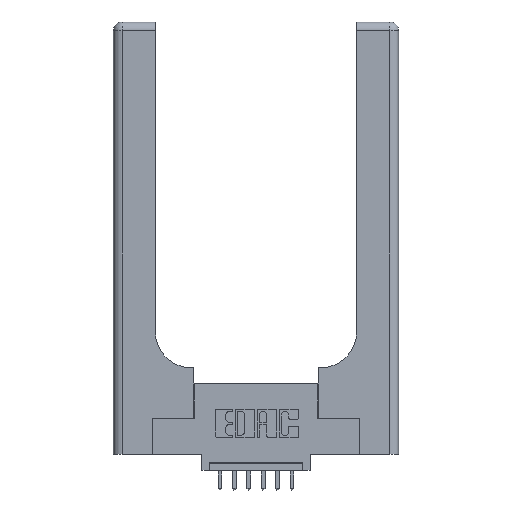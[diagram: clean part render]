
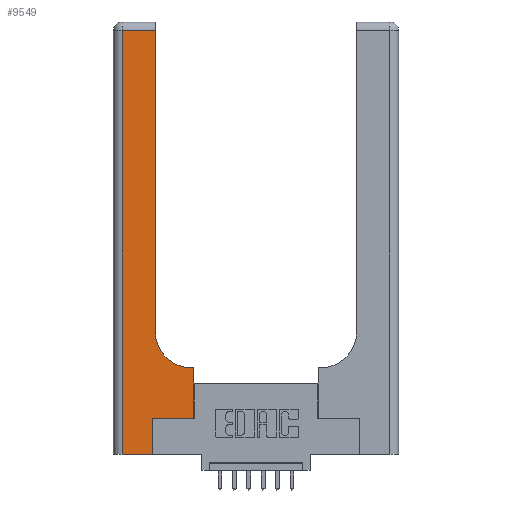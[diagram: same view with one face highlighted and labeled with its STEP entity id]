
A CAD part, top view. The second image highlights one B-rep face of the part: STEP entity #9549.
In plain terms, the highlighted planar face has unit normal (0, 0, 1).
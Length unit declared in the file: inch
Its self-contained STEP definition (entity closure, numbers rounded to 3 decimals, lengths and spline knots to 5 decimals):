
#137 = CARTESIAN_POINT ( 'NONE',  ( 0.5415, 0.85, 0.37 ) ) ;
#236 = CARTESIAN_POINT ( 'NONE',  ( 0.06, 3., 0.37 ) ) ;
#238 = EDGE_CURVE ( 'NONE', #4879, #9358, #3338, .T. ) ;
#274 = DIRECTION ( 'NONE',  ( 0., 1., 0. ) ) ;
#506 = LINE ( 'NONE', #9152, #2619 ) ;
#515 = EDGE_CURVE ( 'NONE', #2527, #6985, #2794, .T. ) ;
#614 = DIRECTION ( 'NONE',  ( -1., 0., 0. ) ) ;
#635 = LINE ( 'NONE', #14375, #2050 ) ;
#674 = DIRECTION ( 'NONE',  ( -1., 0., 0. ) ) ;
#1168 = CARTESIAN_POINT ( 'NONE',  ( 0.2915, 2.94, 0.37 ) ) ;
#1397 = CARTESIAN_POINT ( 'NONE',  ( 0.2915, 3., 0.37 ) ) ;
#1679 = ORIENTED_EDGE ( 'NONE', *, *, #5510, .T. ) ;
#1948 = ORIENTED_EDGE ( 'NONE', *, *, #238, .T. ) ;
#2050 = VECTOR ( 'NONE', #674, 39.37008 ) ;
#2288 = VERTEX_POINT ( 'NONE', #5535 ) ;
#2420 = VECTOR ( 'NONE', #274, 39.37008 ) ;
#2527 = VERTEX_POINT ( 'NONE', #14128 ) ;
#2609 = VECTOR ( 'NONE', #11451, 39.37008 ) ;
#2619 = VECTOR ( 'NONE', #3459, 39.37008 ) ;
#2646 = CARTESIAN_POINT ( 'NONE',  ( 0.269, 0.25, 0.37 ) ) ;
#2728 = CARTESIAN_POINT ( 'NONE',  ( 0.2915, 0.6, 0.37 ) ) ;
#2794 = LINE ( 'NONE', #1397, #2420 ) ;
#3338 = LINE ( 'NONE', #236, #2609 ) ;
#3459 = DIRECTION ( 'NONE',  ( 1., 0., 0. ) ) ;
#3832 = DIRECTION ( 'NONE',  ( -1., 0., 0. ) ) ;
#4016 = EDGE_CURVE ( 'NONE', #4122, #7114, #7437, .T. ) ;
#4049 = EDGE_CURVE ( 'NONE', #7114, #7739, #4609, .T. ) ;
#4122 = VERTEX_POINT ( 'NONE', #6364 ) ;
#4609 = LINE ( 'NONE', #2646, #12596 ) ;
#4657 = FACE_OUTER_BOUND ( 'NONE', #4979, .T. ) ;
#4826 = EDGE_CURVE ( 'NONE', #9358, #4122, #506, .T. ) ;
#4871 = CARTESIAN_POINT ( 'NONE',  ( 0.5585, 0.25, 0.37 ) ) ;
#4879 = VERTEX_POINT ( 'NONE', #6829 ) ;
#4979 = EDGE_LOOP ( 'NONE', ( #12961, #14615, #1948, #8082, #6424, #6780, #1679, #11192, #9993 ) ) ;
#5103 = LINE ( 'NONE', #4871, #8466 ) ;
#5209 = CIRCLE ( 'NONE', #8285, 0.25 ) ;
#5510 = EDGE_CURVE ( 'NONE', #7739, #9836, #5103, .T. ) ;
#5535 = CARTESIAN_POINT ( 'NONE',  ( 0.5415, 0.6, 0.37 ) ) ;
#6364 = CARTESIAN_POINT ( 'NONE',  ( 0.269, 0., 0.37 ) ) ;
#6424 = ORIENTED_EDGE ( 'NONE', *, *, #4016, .T. ) ;
#6780 = ORIENTED_EDGE ( 'NONE', *, *, #4049, .T. ) ;
#6829 = CARTESIAN_POINT ( 'NONE',  ( 0.06, 2.94, 0.37 ) ) ;
#6864 = CARTESIAN_POINT ( 'NONE',  ( 0.5585, 0.6, 0.37 ) ) ;
#6985 = VERTEX_POINT ( 'NONE', #1168 ) ;
#7079 = VECTOR ( 'NONE', #11590, 39.37008 ) ;
#7101 = DIRECTION ( 'NONE',  ( 0., 1., 0. ) ) ;
#7103 = LINE ( 'NONE', #2728, #12258 ) ;
#7114 = VERTEX_POINT ( 'NONE', #10440 ) ;
#7437 = LINE ( 'NONE', #12838, #7079 ) ;
#7444 = EDGE_CURVE ( 'NONE', #6985, #4879, #635, .T. ) ;
#7595 = PLANE ( 'NONE',  #8007 ) ;
#7739 = VERTEX_POINT ( 'NONE', #12479 ) ;
#8007 = AXIS2_PLACEMENT_3D ( 'NONE', #14362, #14409, #614 ) ;
#8082 = ORIENTED_EDGE ( 'NONE', *, *, #4826, .T. ) ;
#8285 = AXIS2_PLACEMENT_3D ( 'NONE', #137, #9202, #10359 ) ;
#8466 = VECTOR ( 'NONE', #7101, 39.37008 ) ;
#8974 = EDGE_CURVE ( 'NONE', #2288, #2527, #5209, .T. ) ;
#9152 = CARTESIAN_POINT ( 'NONE',  ( 0., 0., 0.37 ) ) ;
#9202 = DIRECTION ( 'NONE',  ( 0., 0., -1. ) ) ;
#9293 = CARTESIAN_POINT ( 'NONE',  ( 0.06, 0., 0.37 ) ) ;
#9358 = VERTEX_POINT ( 'NONE', #9293 ) ;
#9549 = ADVANCED_FACE ( 'NONE', ( #4657 ), #7595, .F. ) ;
#9836 = VERTEX_POINT ( 'NONE', #6864 ) ;
#9993 = ORIENTED_EDGE ( 'NONE', *, *, #8974, .T. ) ;
#10359 = DIRECTION ( 'NONE',  ( 1., 0., 0. ) ) ;
#10440 = CARTESIAN_POINT ( 'NONE',  ( 0.269, 0.25, 0.37 ) ) ;
#10508 = EDGE_CURVE ( 'NONE', #9836, #2288, #7103, .T. ) ;
#10602 = DIRECTION ( 'NONE',  ( 1., 0., 0. ) ) ;
#11192 = ORIENTED_EDGE ( 'NONE', *, *, #10508, .T. ) ;
#11451 = DIRECTION ( 'NONE',  ( 0., -1., 0. ) ) ;
#11590 = DIRECTION ( 'NONE',  ( 0., 1., 0. ) ) ;
#12258 = VECTOR ( 'NONE', #3832, 39.37008 ) ;
#12479 = CARTESIAN_POINT ( 'NONE',  ( 0.5585, 0.25, 0.37 ) ) ;
#12596 = VECTOR ( 'NONE', #10602, 39.37008 ) ;
#12838 = CARTESIAN_POINT ( 'NONE',  ( 0.269, 0., 0.37 ) ) ;
#12961 = ORIENTED_EDGE ( 'NONE', *, *, #515, .T. ) ;
#14128 = CARTESIAN_POINT ( 'NONE',  ( 0.2915, 0.85, 0.37 ) ) ;
#14362 = CARTESIAN_POINT ( 'NONE',  ( 0., 3., 0.37 ) ) ;
#14375 = CARTESIAN_POINT ( 'NONE',  ( 0., 2.94, 0.37 ) ) ;
#14409 = DIRECTION ( 'NONE',  ( 0., 0., -1. ) ) ;
#14615 = ORIENTED_EDGE ( 'NONE', *, *, #7444, .T. ) ;
